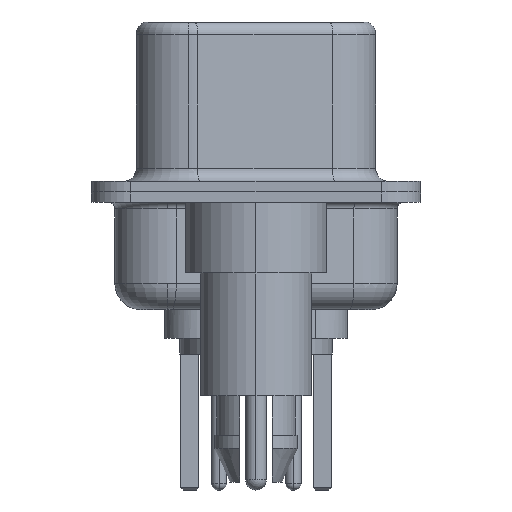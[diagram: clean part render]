
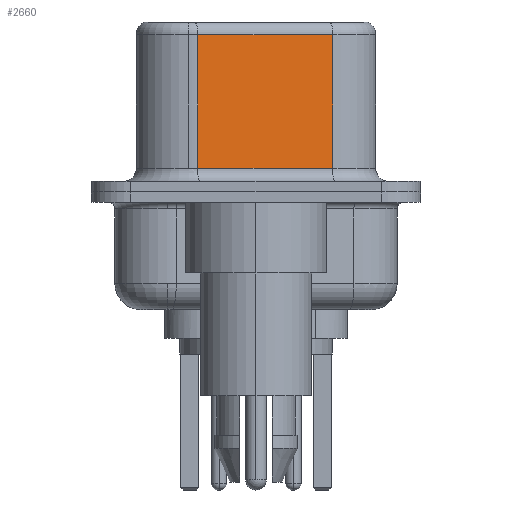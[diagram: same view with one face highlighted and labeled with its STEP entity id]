
A CAD part, left-side view. The second image highlights one B-rep face of the part: STEP entity #2660.
In plain terms, the highlighted planar face has unit normal (-0.985, -0.174, 0).
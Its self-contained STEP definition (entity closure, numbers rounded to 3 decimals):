
#421 = CARTESIAN_POINT ( 'NONE',  ( 4.585, -2.927, 6.02 ) ) ;
#454 = CARTESIAN_POINT ( 'NONE',  ( 3.675, 2.233, 0.9 ) ) ;
#635 = ORIENTED_EDGE ( 'NONE', *, *, #3604, .F. ) ;
#767 = DIRECTION ( 'NONE',  ( 0.174, -0.985, 0. ) ) ;
#819 = DIRECTION ( 'NONE',  ( -0.174, 0.985, 0. ) ) ;
#934 = VECTOR ( 'NONE', #8732, 1000. ) ;
#1283 = DIRECTION ( 'NONE',  ( 0.985, 0.174, 0. ) ) ;
#2011 = VERTEX_POINT ( 'NONE', #14974 ) ;
#2660 = ADVANCED_FACE ( 'NONE', ( #14061 ), #6799, .F. ) ;
#3354 = DIRECTION ( 'NONE',  ( 0., 0., -1. ) ) ;
#3604 = EDGE_CURVE ( 'NONE', #5974, #5126, #12257, .T. ) ;
#4902 = VECTOR ( 'NONE', #819, 1000. ) ;
#5126 = VERTEX_POINT ( 'NONE', #17867 ) ;
#5329 = AXIS2_PLACEMENT_3D ( 'NONE', #11789, #1283, #11763 ) ;
#5928 = EDGE_CURVE ( 'NONE', #5974, #2011, #13430, .T. ) ;
#5974 = VERTEX_POINT ( 'NONE', #15062 ) ;
#6461 = VECTOR ( 'NONE', #767, 1000. ) ;
#6693 = EDGE_CURVE ( 'NONE', #2011, #19928, #13661, .T. ) ;
#6799 = PLANE ( 'NONE',  #5329 ) ;
#7187 = CARTESIAN_POINT ( 'NONE',  ( 4.585, -2.927, 6.52 ) ) ;
#8732 = DIRECTION ( 'NONE',  ( 0., 0., -1. ) ) ;
#10201 = CARTESIAN_POINT ( 'NONE',  ( 3.675, 2.233, 6.52 ) ) ;
#11071 = EDGE_CURVE ( 'NONE', #19928, #5126, #19326, .T. ) ;
#11763 = DIRECTION ( 'NONE',  ( -0.174, 0.985, 0. ) ) ;
#11789 = CARTESIAN_POINT ( 'NONE',  ( 4.585, -2.927, 6.52 ) ) ;
#12257 = LINE ( 'NONE', #7187, #16041 ) ;
#12453 = ORIENTED_EDGE ( 'NONE', *, *, #5928, .T. ) ;
#13430 = LINE ( 'NONE', #421, #4902 ) ;
#13603 = ORIENTED_EDGE ( 'NONE', *, *, #11071, .T. ) ;
#13661 = LINE ( 'NONE', #10201, #934 ) ;
#14061 = FACE_OUTER_BOUND ( 'NONE', #15628, .T. ) ;
#14291 = ORIENTED_EDGE ( 'NONE', *, *, #6693, .T. ) ;
#14974 = CARTESIAN_POINT ( 'NONE',  ( 3.675, 2.233, 6.02 ) ) ;
#15062 = CARTESIAN_POINT ( 'NONE',  ( 4.585, -2.927, 6.02 ) ) ;
#15628 = EDGE_LOOP ( 'NONE', ( #635, #12453, #14291, #13603 ) ) ;
#16041 = VECTOR ( 'NONE', #3354, 1000. ) ;
#17867 = CARTESIAN_POINT ( 'NONE',  ( 4.585, -2.927, 0.9 ) ) ;
#19326 = LINE ( 'NONE', #19897, #6461 ) ;
#19897 = CARTESIAN_POINT ( 'NONE',  ( 4.585, -2.927, 0.9 ) ) ;
#19928 = VERTEX_POINT ( 'NONE', #454 ) ;
